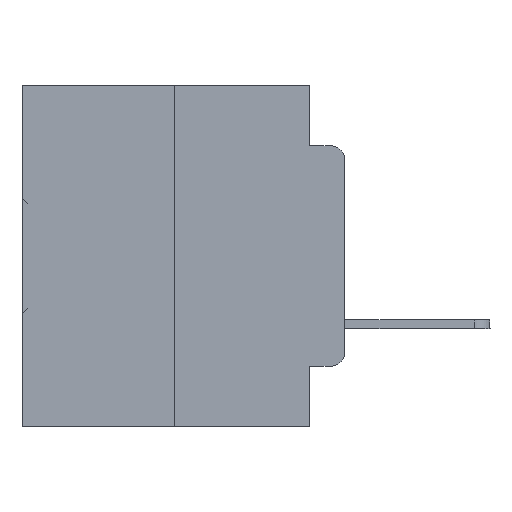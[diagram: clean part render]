
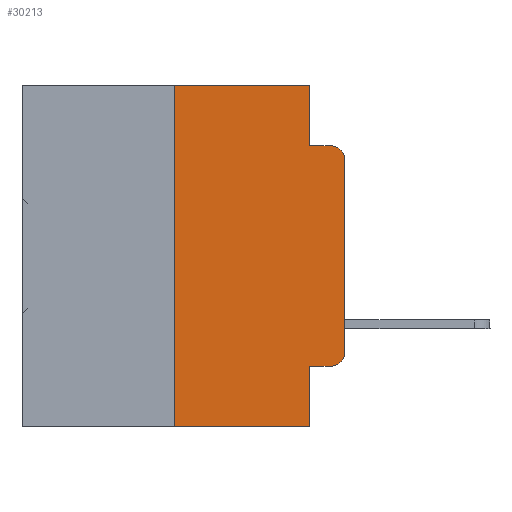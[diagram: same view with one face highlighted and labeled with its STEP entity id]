
A CAD part, left-side view. The second image highlights one B-rep face of the part: STEP entity #30213.
In plain terms, the highlighted planar face has unit normal (-1, 0, 0).
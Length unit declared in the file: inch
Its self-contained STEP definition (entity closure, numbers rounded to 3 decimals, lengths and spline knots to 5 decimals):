
#114 = DIRECTION ( 'NONE',  ( -1., 0., 0. ) ) ;
#1323 = VERTEX_POINT ( 'NONE', #30081 ) ;
#1662 = VERTEX_POINT ( 'NONE', #28393 ) ;
#1722 = VERTEX_POINT ( 'NONE', #21282 ) ;
#1781 = EDGE_CURVE ( 'NONE', #15448, #3551, #5869, .T. ) ;
#2247 = CARTESIAN_POINT ( 'NONE',  ( 0., 0.25, -0.5 ) ) ;
#2734 = CARTESIAN_POINT ( 'NONE',  ( 0., 0.473, -0.5 ) ) ;
#2974 = ORIENTED_EDGE ( 'NONE', *, *, #12443, .T. ) ;
#3397 = LINE ( 'NONE', #22398, #28177 ) ;
#3551 = VERTEX_POINT ( 'NONE', #26734 ) ;
#3629 = DIRECTION ( 'NONE',  ( 0., 0., -1. ) ) ;
#3980 = ORIENTED_EDGE ( 'NONE', *, *, #21084, .T. ) ;
#4243 = LINE ( 'NONE', #24841, #6710 ) ;
#4394 = ORIENTED_EDGE ( 'NONE', *, *, #20146, .F. ) ;
#4747 = LINE ( 'NONE', #33658, #17982 ) ;
#4775 = DIRECTION ( 'NONE',  ( 0., 0., -1. ) ) ;
#5211 = EDGE_CURVE ( 'NONE', #15448, #28984, #7898, .T. ) ;
#5397 = LINE ( 'NONE', #28182, #25658 ) ;
#5531 = EDGE_CURVE ( 'NONE', #6306, #30136, #5397, .T. ) ;
#5869 = LINE ( 'NONE', #2734, #15786 ) ;
#6087 = VECTOR ( 'NONE', #26812, 39.37008 ) ;
#6306 = VERTEX_POINT ( 'NONE', #25738 ) ;
#6360 = CARTESIAN_POINT ( 'NONE',  ( 0., 0., -0.1085 ) ) ;
#6710 = VECTOR ( 'NONE', #9257, 39.37008 ) ;
#6874 = ORIENTED_EDGE ( 'NONE', *, *, #10639, .T. ) ;
#7152 = AXIS2_PLACEMENT_3D ( 'NONE', #30152, #32698, #3629 ) ;
#7364 = CARTESIAN_POINT ( 'NONE',  ( 0., 0.25, 0. ) ) ;
#7898 = LINE ( 'NONE', #7364, #14545 ) ;
#7968 = CARTESIAN_POINT ( 'NONE',  ( 0., 0.02, -0.4115 ) ) ;
#8913 = PLANE ( 'NONE',  #28121 ) ;
#9187 = EDGE_CURVE ( 'NONE', #1722, #3551, #4747, .T. ) ;
#9257 = DIRECTION ( 'NONE',  ( 0., 0., 1. ) ) ;
#9610 = CIRCLE ( 'NONE', #13765, 0.02 ) ;
#10042 = DIRECTION ( 'NONE',  ( 0., 0., 1. ) ) ;
#10639 = EDGE_CURVE ( 'NONE', #1323, #20816, #4243, .T. ) ;
#10767 = ORIENTED_EDGE ( 'NONE', *, *, #1781, .T. ) ;
#12443 = EDGE_CURVE ( 'NONE', #26125, #1323, #23146, .T. ) ;
#13765 = AXIS2_PLACEMENT_3D ( 'NONE', #28729, #114, #33936 ) ;
#14545 = VECTOR ( 'NONE', #10042, 39.37008 ) ;
#14584 = ORIENTED_EDGE ( 'NONE', *, *, #5531, .F. ) ;
#15448 = VERTEX_POINT ( 'NONE', #2247 ) ;
#15531 = EDGE_LOOP ( 'NONE', ( #6874, #3980, #4394, #14584, #26524, #20737, #10767, #27344, #23763, #2974 ) ) ;
#15786 = VECTOR ( 'NONE', #21551, 39.37008 ) ;
#16396 = EDGE_CURVE ( 'NONE', #1722, #26125, #22977, .T. ) ;
#16772 = CARTESIAN_POINT ( 'NONE',  ( 0., 0.473, 0. ) ) ;
#17982 = VECTOR ( 'NONE', #4775, 39.37008 ) ;
#19460 = DIRECTION ( 'NONE',  ( 1., 0., 0. ) ) ;
#20146 = EDGE_CURVE ( 'NONE', #30136, #1662, #20169, .T. ) ;
#20169 = LINE ( 'NONE', #30275, #6087 ) ;
#20429 = FACE_OUTER_BOUND ( 'NONE', #15531, .T. ) ;
#20737 = ORIENTED_EDGE ( 'NONE', *, *, #5211, .F. ) ;
#20816 = VERTEX_POINT ( 'NONE', #6360 ) ;
#21084 = EDGE_CURVE ( 'NONE', #20816, #1662, #9610, .T. ) ;
#21147 = EDGE_CURVE ( 'NONE', #28984, #6306, #3397, .T. ) ;
#21282 = CARTESIAN_POINT ( 'NONE',  ( 0., 0.051, -0.4115 ) ) ;
#21551 = DIRECTION ( 'NONE',  ( 0., -1., 0. ) ) ;
#22225 = DIRECTION ( 'NONE',  ( 0., 0., -1. ) ) ;
#22398 = CARTESIAN_POINT ( 'NONE',  ( 0., 0.473, 0. ) ) ;
#22441 = CARTESIAN_POINT ( 'NONE',  ( 0., 0.051, -0.4115 ) ) ;
#22799 = DIRECTION ( 'NONE',  ( 0., 0., -1. ) ) ;
#22977 = LINE ( 'NONE', #22441, #32421 ) ;
#23146 = CIRCLE ( 'NONE', #7152, 0.02 ) ;
#23763 = ORIENTED_EDGE ( 'NONE', *, *, #16396, .T. ) ;
#24841 = CARTESIAN_POINT ( 'NONE',  ( 0., 0., 0. ) ) ;
#25658 = VECTOR ( 'NONE', #22799, 39.37008 ) ;
#25738 = CARTESIAN_POINT ( 'NONE',  ( 0., 0.051, 0. ) ) ;
#26125 = VERTEX_POINT ( 'NONE', #7968 ) ;
#26524 = ORIENTED_EDGE ( 'NONE', *, *, #21147, .F. ) ;
#26734 = CARTESIAN_POINT ( 'NONE',  ( 0., 0.051, -0.5 ) ) ;
#26812 = DIRECTION ( 'NONE',  ( 0., -1., 0. ) ) ;
#27344 = ORIENTED_EDGE ( 'NONE', *, *, #9187, .F. ) ;
#28121 = AXIS2_PLACEMENT_3D ( 'NONE', #16772, #19460, #22225 ) ;
#28177 = VECTOR ( 'NONE', #32796, 39.37008 ) ;
#28182 = CARTESIAN_POINT ( 'NONE',  ( 0., 0.051, 0. ) ) ;
#28393 = CARTESIAN_POINT ( 'NONE',  ( 0., 0.02, -0.0885 ) ) ;
#28523 = DIRECTION ( 'NONE',  ( 0., -1., 0. ) ) ;
#28729 = CARTESIAN_POINT ( 'NONE',  ( 0., 0.02, -0.1085 ) ) ;
#28984 = VERTEX_POINT ( 'NONE', #33141 ) ;
#30081 = CARTESIAN_POINT ( 'NONE',  ( 0., 0., -0.3915 ) ) ;
#30136 = VERTEX_POINT ( 'NONE', #32359 ) ;
#30152 = CARTESIAN_POINT ( 'NONE',  ( 0., 0.02, -0.3915 ) ) ;
#30213 = ADVANCED_FACE ( 'NONE', ( #20429 ), #8913, .F. ) ;
#30275 = CARTESIAN_POINT ( 'NONE',  ( 0., 0.051, -0.0885 ) ) ;
#32359 = CARTESIAN_POINT ( 'NONE',  ( 0., 0.051, -0.0885 ) ) ;
#32421 = VECTOR ( 'NONE', #28523, 39.37008 ) ;
#32698 = DIRECTION ( 'NONE',  ( -1., 0., 0. ) ) ;
#32796 = DIRECTION ( 'NONE',  ( 0., -1., 0. ) ) ;
#33141 = CARTESIAN_POINT ( 'NONE',  ( 0., 0.25, 0. ) ) ;
#33658 = CARTESIAN_POINT ( 'NONE',  ( 0., 0.051, 0. ) ) ;
#33936 = DIRECTION ( 'NONE',  ( 0., 0., -1. ) ) ;
